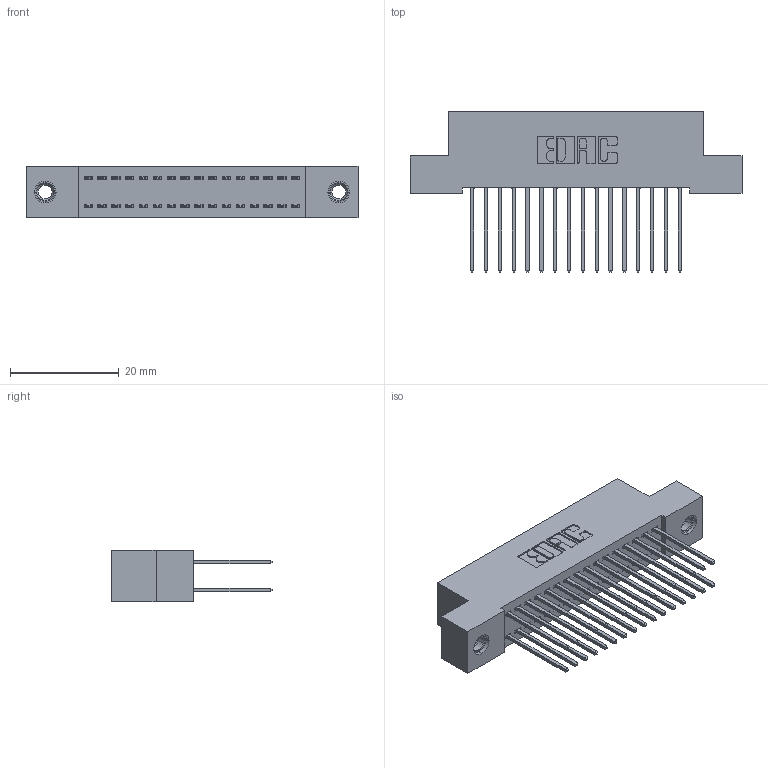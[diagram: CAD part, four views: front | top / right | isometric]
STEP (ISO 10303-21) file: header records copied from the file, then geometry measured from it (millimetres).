
FILE_DESCRIPTION (( 'STEP AP203' ), '1' );
FILE_NAME ('342-032-540-207.STEP', '2018-08-11T16:57:23', ( '' ), ( '' ), 'SwSTEP 2.0', 'SolidWorks 2016', '' );
FILE_SCHEMA (( 'CONFIG_CONTROL_DESIGN' ));
Length unit declared in the file: inch
Products named in the file (4): 345-292-001_345-293-140; 345-250-001_345-250-005-103; 342-032-540-207; 342 Part_TI
Assembly tree (35 placements, depth 2):
  342-032-540-207
    342 Part_TI
    345-292-001_345-293-140  x32
    345-250-001_345-250-005-103  x2
Bounding box: 60.96 x 29.47 x 9.4 mm (x, y, z)
Volume: 5462.8 mm3; surface area: 8816.5 mm2
Topology: 35 solids, 35 shells, 1834 faces, 5395 edges, 3546 vertices
Faces by surface type: plane 1250, cylinder 568, cone 12, torus 4
Entity records: 14728 total; most frequent: CARTESIAN_POINT 2453, ORIENTED_EDGE 2382, DIRECTION 2173, EDGE_CURVE 1191, VECTOR 1043, LINE 1043, VERTEX_POINT 788, AXIS2_PLACEMENT_3D 565
